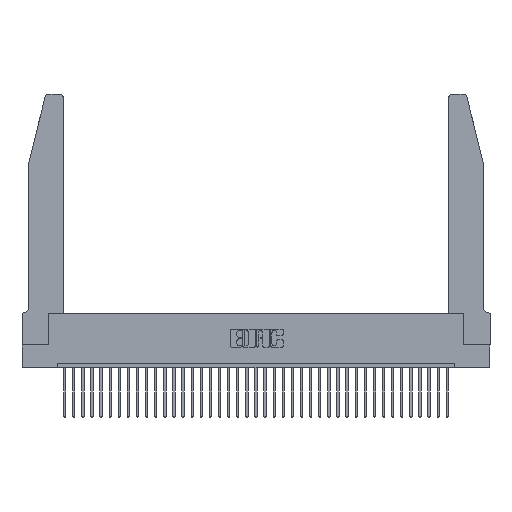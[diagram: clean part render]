
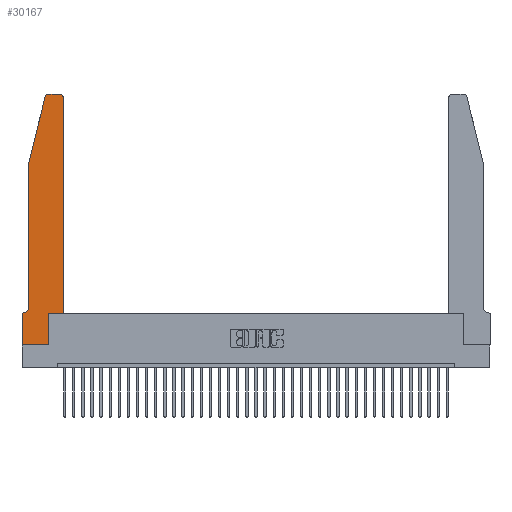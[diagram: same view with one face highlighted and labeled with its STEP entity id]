
A CAD part, top view. The second image highlights one B-rep face of the part: STEP entity #30167.
In plain terms, the highlighted planar face has unit normal (0, 0, 1).
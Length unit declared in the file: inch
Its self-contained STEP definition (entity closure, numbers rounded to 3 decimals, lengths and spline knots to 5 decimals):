
#33 = VECTOR ( 'NONE', #459, 39.37008 ) ;
#449 = VERTEX_POINT ( 'NONE', #22386 ) ;
#459 = DIRECTION ( 'NONE',  ( 1., 0., 0. ) ) ;
#596 = VERTEX_POINT ( 'NONE', #10233 ) ;
#698 = ORIENTED_EDGE ( 'NONE', *, *, #5901, .T. ) ;
#1377 = CARTESIAN_POINT ( 'NONE',  ( 0., 0.35, 0.37 ) ) ;
#1840 = VECTOR ( 'NONE', #21660, 39.37008 ) ;
#2085 = DIRECTION ( 'NONE',  ( 0., -1., 0. ) ) ;
#2448 = LINE ( 'NONE', #19189, #17226 ) ;
#3200 = CARTESIAN_POINT ( 'NONE',  ( 0.284, 2.72, 0.37 ) ) ;
#3243 = LINE ( 'NONE', #8007, #34971 ) ;
#4295 = ORIENTED_EDGE ( 'NONE', *, *, #16596, .T. ) ;
#4495 = LINE ( 'NONE', #33034, #1840 ) ;
#4746 = AXIS2_PLACEMENT_3D ( 'NONE', #1377, #32752, #9633 ) ;
#5194 = VERTEX_POINT ( 'NONE', #16837 ) ;
#5837 = CARTESIAN_POINT ( 'NONE',  ( 0., 0., 0.37 ) ) ;
#5901 = EDGE_CURVE ( 'NONE', #26920, #33801, #24626, .T. ) ;
#6064 = CIRCLE ( 'NONE', #19666, 0.07 ) ;
#6283 = ORIENTED_EDGE ( 'NONE', *, *, #29540, .T. ) ;
#6302 = DIRECTION ( 'NONE',  ( 0., 0., 1. ) ) ;
#7262 = EDGE_CURVE ( 'NONE', #31552, #596, #4495, .T. ) ;
#7758 = FACE_OUTER_BOUND ( 'NONE', #10211, .T. ) ;
#7984 = DIRECTION ( 'NONE',  ( 0., 1., 0. ) ) ;
#8007 = CARTESIAN_POINT ( 'NONE',  ( 0.2605, 2.75, 0.37 ) ) ;
#8280 = DIRECTION ( 'NONE',  ( 0., -1., 0. ) ) ;
#8879 = CARTESIAN_POINT ( 'NONE',  ( 0.284, 2.75, 0.37 ) ) ;
#8928 = EDGE_CURVE ( 'NONE', #33801, #20792, #36974, .T. ) ;
#9089 = CARTESIAN_POINT ( 'NONE',  ( 0.0755, 0.35, 0.37 ) ) ;
#9141 = CARTESIAN_POINT ( 'NONE',  ( 0., 0., 0.37 ) ) ;
#9633 = DIRECTION ( 'NONE',  ( 1., 0., 0. ) ) ;
#9646 = ORIENTED_EDGE ( 'NONE', *, *, #12832, .T. ) ;
#9647 = EDGE_CURVE ( 'NONE', #12723, #5194, #31131, .T. ) ;
#10058 = CARTESIAN_POINT ( 'NONE',  ( 0.4205, 2.72, 0.37 ) ) ;
#10166 = LINE ( 'NONE', #9089, #14681 ) ;
#10211 = EDGE_LOOP ( 'NONE', ( #26031, #31661, #17189, #15099, #18726, #9646, #4295, #698, #27908, #30469, #21994, #6283 ) ) ;
#10233 = CARTESIAN_POINT ( 'NONE',  ( 0.4505, 2.72, 0.37 ) ) ;
#10636 = CARTESIAN_POINT ( 'NONE',  ( 0.2865, 0.35, 0.37 ) ) ;
#10979 = DIRECTION ( 'NONE',  ( 0., 0., -1. ) ) ;
#11366 = CARTESIAN_POINT ( 'NONE',  ( 0.0055, 0.35, 0.37 ) ) ;
#11763 = VERTEX_POINT ( 'NONE', #11366 ) ;
#12077 = LINE ( 'NONE', #26265, #19677 ) ;
#12723 = VERTEX_POINT ( 'NONE', #32325 ) ;
#12832 = EDGE_CURVE ( 'NONE', #11763, #31452, #10166, .T. ) ;
#14367 = DIRECTION ( 'NONE',  ( -1., 0., 0. ) ) ;
#14651 = CARTESIAN_POINT ( 'NONE',  ( 0.0755, 0.42, 0.37 ) ) ;
#14681 = VECTOR ( 'NONE', #34807, 39.37008 ) ;
#15099 = ORIENTED_EDGE ( 'NONE', *, *, #22134, .T. ) ;
#16197 = VERTEX_POINT ( 'NONE', #8879 ) ;
#16596 = EDGE_CURVE ( 'NONE', #31452, #26920, #26413, .T. ) ;
#16837 = CARTESIAN_POINT ( 'NONE',  ( 0.0755, 2., 0.37 ) ) ;
#16993 = CIRCLE ( 'NONE', #22443, 0.03 ) ;
#17189 = ORIENTED_EDGE ( 'NONE', *, *, #9647, .T. ) ;
#17226 = VECTOR ( 'NONE', #2085, 39.37008 ) ;
#18019 = EDGE_CURVE ( 'NONE', #16197, #12723, #16993, .T. ) ;
#18449 = CARTESIAN_POINT ( 'NONE',  ( 0.4505, 0.35, 0.37 ) ) ;
#18533 = CIRCLE ( 'NONE', #20969, 0.03 ) ;
#18726 = ORIENTED_EDGE ( 'NONE', *, *, #33802, .T. ) ;
#19135 = EDGE_CURVE ( 'NONE', #20792, #31552, #12077, .T. ) ;
#19189 = CARTESIAN_POINT ( 'NONE',  ( 0.0755, 2., 0.37 ) ) ;
#19633 = CARTESIAN_POINT ( 'NONE',  ( 0., 0., 0.37 ) ) ;
#19666 = AXIS2_PLACEMENT_3D ( 'NONE', #20054, #10979, #14367 ) ;
#19677 = VECTOR ( 'NONE', #32249, 39.37008 ) ;
#19942 = CARTESIAN_POINT ( 'NONE',  ( 0.2865, 0., 0.37 ) ) ;
#20054 = CARTESIAN_POINT ( 'NONE',  ( 0.0055, 0.42, 0.37 ) ) ;
#20792 = VERTEX_POINT ( 'NONE', #36924 ) ;
#20969 = AXIS2_PLACEMENT_3D ( 'NONE', #10058, #27565, #24153 ) ;
#21660 = DIRECTION ( 'NONE',  ( 0., 1., 0. ) ) ;
#21994 = ORIENTED_EDGE ( 'NONE', *, *, #7262, .T. ) ;
#22134 = EDGE_CURVE ( 'NONE', #5194, #28722, #2448, .T. ) ;
#22386 = CARTESIAN_POINT ( 'NONE',  ( 0.4205, 2.75, 0.37 ) ) ;
#22443 = AXIS2_PLACEMENT_3D ( 'NONE', #3200, #6302, #26215 ) ;
#23831 = CARTESIAN_POINT ( 'NONE',  ( 0.0755, 2., 0.37 ) ) ;
#24153 = DIRECTION ( 'NONE',  ( 1., 0., 0. ) ) ;
#24626 = LINE ( 'NONE', #5837, #33 ) ;
#25396 = VECTOR ( 'NONE', #7984, 39.37008 ) ;
#26031 = ORIENTED_EDGE ( 'NONE', *, *, #30431, .T. ) ;
#26082 = CARTESIAN_POINT ( 'NONE',  ( 0., 0.35, 0.37 ) ) ;
#26215 = DIRECTION ( 'NONE',  ( 1., 0., 0. ) ) ;
#26265 = CARTESIAN_POINT ( 'NONE',  ( 0.4505, 0.35, 0.37 ) ) ;
#26413 = LINE ( 'NONE', #19633, #34878 ) ;
#26920 = VERTEX_POINT ( 'NONE', #9141 ) ;
#27565 = DIRECTION ( 'NONE',  ( 0., 0., 1. ) ) ;
#27908 = ORIENTED_EDGE ( 'NONE', *, *, #8928, .T. ) ;
#28722 = VERTEX_POINT ( 'NONE', #14651 ) ;
#29540 = EDGE_CURVE ( 'NONE', #596, #449, #18533, .T. ) ;
#29550 = DIRECTION ( 'NONE',  ( -0.239, -0.971, 0. ) ) ;
#30167 = ADVANCED_FACE ( 'NONE', ( #7758 ), #35597, .T. ) ;
#30431 = EDGE_CURVE ( 'NONE', #449, #16197, #3243, .T. ) ;
#30469 = ORIENTED_EDGE ( 'NONE', *, *, #19135, .T. ) ;
#31131 = LINE ( 'NONE', #23831, #32018 ) ;
#31452 = VERTEX_POINT ( 'NONE', #26082 ) ;
#31552 = VERTEX_POINT ( 'NONE', #18449 ) ;
#31661 = ORIENTED_EDGE ( 'NONE', *, *, #18019, .T. ) ;
#32018 = VECTOR ( 'NONE', #29550, 39.37008 ) ;
#32249 = DIRECTION ( 'NONE',  ( 1., 0., 0. ) ) ;
#32325 = CARTESIAN_POINT ( 'NONE',  ( 0.25487, 2.72718, 0.37 ) ) ;
#32752 = DIRECTION ( 'NONE',  ( 0., 0., 1. ) ) ;
#33034 = CARTESIAN_POINT ( 'NONE',  ( 0.4505, 0.35, 0.37 ) ) ;
#33801 = VERTEX_POINT ( 'NONE', #19942 ) ;
#33802 = EDGE_CURVE ( 'NONE', #28722, #11763, #6064, .T. ) ;
#34807 = DIRECTION ( 'NONE',  ( -1., 0., 0. ) ) ;
#34878 = VECTOR ( 'NONE', #8280, 39.37008 ) ;
#34971 = VECTOR ( 'NONE', #36349, 39.37008 ) ;
#35597 = PLANE ( 'NONE',  #4746 ) ;
#36349 = DIRECTION ( 'NONE',  ( -1., 0., 0. ) ) ;
#36924 = CARTESIAN_POINT ( 'NONE',  ( 0.2865, 0.35, 0.37 ) ) ;
#36974 = LINE ( 'NONE', #10636, #25396 ) ;
